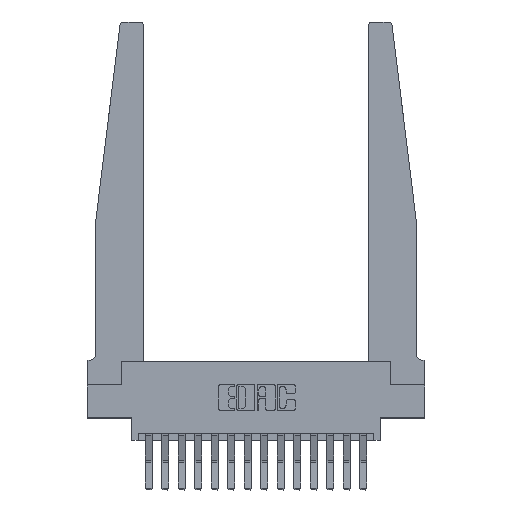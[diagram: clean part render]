
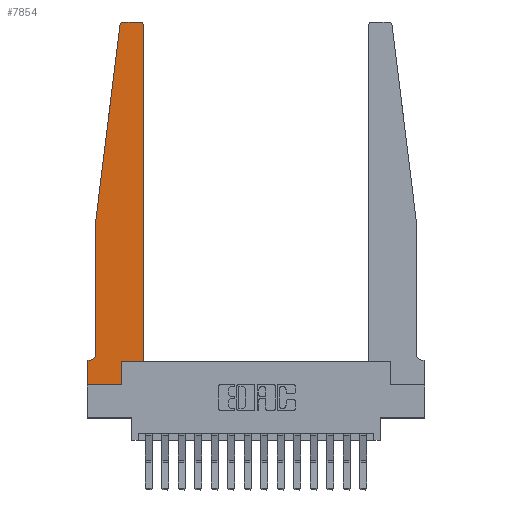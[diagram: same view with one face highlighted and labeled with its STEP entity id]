
A CAD part, top view. The second image highlights one B-rep face of the part: STEP entity #7854.
In plain terms, the highlighted planar face has unit normal (0, 0, 1).
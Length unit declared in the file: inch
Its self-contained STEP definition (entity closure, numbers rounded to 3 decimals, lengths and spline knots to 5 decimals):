
#316 = VERTEX_POINT ( 'NONE', #14830 ) ;
#393 = ORIENTED_EDGE ( 'NONE', *, *, #10516, .T. ) ;
#430 = AXIS2_PLACEMENT_3D ( 'NONE', #8690, #3119, #10266 ) ;
#656 = LINE ( 'NONE', #6327, #4585 ) ;
#957 = DIRECTION ( 'NONE',  ( 0., 1., 0. ) ) ;
#1023 = LINE ( 'NONE', #9667, #18153 ) ;
#1343 = VECTOR ( 'NONE', #957, 39.37008 ) ;
#1388 = EDGE_CURVE ( 'NONE', #12304, #15515, #12120, .T. ) ;
#1461 = DIRECTION ( 'NONE',  ( 0., 0., 1. ) ) ;
#1943 = DIRECTION ( 'NONE',  ( -1., 0., 0. ) ) ;
#2160 = VERTEX_POINT ( 'NONE', #16702 ) ;
#2281 = DIRECTION ( 'NONE',  ( 0., 0., 1. ) ) ;
#2345 = EDGE_CURVE ( 'NONE', #9796, #8731, #17068, .T. ) ;
#2382 = CARTESIAN_POINT ( 'NONE',  ( 0.015, 0.2375, 0.37 ) ) ;
#2872 = DIRECTION ( 'NONE',  ( 0., -1., 0. ) ) ;
#3025 = VERTEX_POINT ( 'NONE', #6925 ) ;
#3119 = DIRECTION ( 'NONE',  ( 0., 0., 1. ) ) ;
#3303 = VECTOR ( 'NONE', #7425, 39.37008 ) ;
#3355 = VECTOR ( 'NONE', #2872, 39.37008 ) ;
#3538 = ORIENTED_EDGE ( 'NONE', *, *, #6006, .T. ) ;
#3960 = EDGE_CURVE ( 'NONE', #8731, #12769, #9577, .T. ) ;
#4111 = ORIENTED_EDGE ( 'NONE', *, *, #2345, .T. ) ;
#4379 = CARTESIAN_POINT ( 'NONE',  ( 0.425, 0.18, 0.37 ) ) ;
#4579 = ORIENTED_EDGE ( 'NONE', *, *, #5078, .T. ) ;
#4585 = VECTOR ( 'NONE', #4944, 39.37008 ) ;
#4708 = EDGE_CURVE ( 'NONE', #18207, #9796, #1023, .T. ) ;
#4944 = DIRECTION ( 'NONE',  ( 0., -1., 0. ) ) ;
#5078 = EDGE_CURVE ( 'NONE', #13765, #14226, #15946, .T. ) ;
#5139 = VECTOR ( 'NONE', #16209, 39.37008 ) ;
#5142 = CARTESIAN_POINT ( 'NONE',  ( 0.2605, 0.18, 0.37 ) ) ;
#5202 = VECTOR ( 'NONE', #1943, 39.37008 ) ;
#5205 = DIRECTION ( 'NONE',  ( 1., 0., 0. ) ) ;
#5713 = ORIENTED_EDGE ( 'NONE', *, *, #1388, .T. ) ;
#5793 = ORIENTED_EDGE ( 'NONE', *, *, #13723, .T. ) ;
#6006 = EDGE_CURVE ( 'NONE', #3025, #12304, #656, .T. ) ;
#6063 = VECTOR ( 'NONE', #16045, 39.37008 ) ;
#6327 = CARTESIAN_POINT ( 'NONE',  ( 0.065, 1.25, 0.37 ) ) ;
#6925 = CARTESIAN_POINT ( 'NONE',  ( 0.065, 1.25, 0.37 ) ) ;
#7110 = ORIENTED_EDGE ( 'NONE', *, *, #15002, .T. ) ;
#7131 = FACE_OUTER_BOUND ( 'NONE', #17316, .T. ) ;
#7241 = EDGE_CURVE ( 'NONE', #14226, #18207, #9322, .T. ) ;
#7381 = ORIENTED_EDGE ( 'NONE', *, *, #7241, .T. ) ;
#7425 = DIRECTION ( 'NONE',  ( 0., 1., 0. ) ) ;
#7524 = VECTOR ( 'NONE', #10487, 39.37008 ) ;
#7686 = CARTESIAN_POINT ( 'NONE',  ( 0.065, 1.25, 0.37 ) ) ;
#7696 = CARTESIAN_POINT ( 'NONE',  ( 0., 0., 0.37 ) ) ;
#7854 = ADVANCED_FACE ( 'NONE', ( #7131 ), #8898, .T. ) ;
#7895 = CARTESIAN_POINT ( 'NONE',  ( 0.425, 2.72, 0.37 ) ) ;
#7953 = DIRECTION ( 'NONE',  ( 1., 0., 0. ) ) ;
#8147 = EDGE_CURVE ( 'NONE', #16716, #2160, #14038, .T. ) ;
#8156 = DIRECTION ( 'NONE',  ( -1., 0., 0. ) ) ;
#8446 = LINE ( 'NONE', #11208, #3355 ) ;
#8533 = CARTESIAN_POINT ( 'NONE',  ( 0., 0.1875, 0.37 ) ) ;
#8690 = CARTESIAN_POINT ( 'NONE',  ( 0.27653, 2.72, 0.37 ) ) ;
#8723 = CARTESIAN_POINT ( 'NONE',  ( 0.27653, 2.75, 0.37 ) ) ;
#8731 = VERTEX_POINT ( 'NONE', #7895 ) ;
#8736 = CARTESIAN_POINT ( 'NONE',  ( 0.065, 0.1875, 0.37 ) ) ;
#8898 = PLANE ( 'NONE',  #17351 ) ;
#9322 = LINE ( 'NONE', #5142, #1343 ) ;
#9577 = CIRCLE ( 'NONE', #12230, 0.03 ) ;
#9667 = CARTESIAN_POINT ( 'NONE',  ( 0.425, 0.18, 0.37 ) ) ;
#9796 = VERTEX_POINT ( 'NONE', #11247 ) ;
#9885 = CARTESIAN_POINT ( 'NONE',  ( 0.065, 0.2375, 0.37 ) ) ;
#10266 = DIRECTION ( 'NONE',  ( 1., 0., 0. ) ) ;
#10487 = DIRECTION ( 'NONE',  ( 1., 0., 0. ) ) ;
#10516 = EDGE_CURVE ( 'NONE', #2160, #3025, #16387, .T. ) ;
#10677 = CARTESIAN_POINT ( 'NONE',  ( 0., 0., 0.37 ) ) ;
#11208 = CARTESIAN_POINT ( 'NONE',  ( 0., 0., 0.37 ) ) ;
#11247 = CARTESIAN_POINT ( 'NONE',  ( 0.425, 0.18, 0.37 ) ) ;
#11561 = EDGE_CURVE ( 'NONE', #316, #13765, #8446, .T. ) ;
#11798 = ORIENTED_EDGE ( 'NONE', *, *, #8147, .T. ) ;
#12120 = CIRCLE ( 'NONE', #15682, 0.05 ) ;
#12219 = DIRECTION ( 'NONE',  ( 0., 0., -1. ) ) ;
#12230 = AXIS2_PLACEMENT_3D ( 'NONE', #14975, #2281, #7953 ) ;
#12304 = VERTEX_POINT ( 'NONE', #9885 ) ;
#12769 = VERTEX_POINT ( 'NONE', #14214 ) ;
#12771 = DIRECTION ( 'NONE',  ( 1., 0., 0. ) ) ;
#13065 = LINE ( 'NONE', #14641, #5202 ) ;
#13723 = EDGE_CURVE ( 'NONE', #15515, #316, #16229, .T. ) ;
#13765 = VERTEX_POINT ( 'NONE', #10677 ) ;
#14038 = CIRCLE ( 'NONE', #430, 0.03 ) ;
#14214 = CARTESIAN_POINT ( 'NONE',  ( 0.395, 2.75, 0.37 ) ) ;
#14226 = VERTEX_POINT ( 'NONE', #15742 ) ;
#14641 = CARTESIAN_POINT ( 'NONE',  ( 0.25, 2.75, 0.37 ) ) ;
#14713 = CARTESIAN_POINT ( 'NONE',  ( 0.015, 0.1875, 0.37 ) ) ;
#14830 = CARTESIAN_POINT ( 'NONE',  ( 0., 0.1875, 0.37 ) ) ;
#14975 = CARTESIAN_POINT ( 'NONE',  ( 0.395, 2.72, 0.37 ) ) ;
#15002 = EDGE_CURVE ( 'NONE', #12769, #16716, #13065, .T. ) ;
#15515 = VERTEX_POINT ( 'NONE', #14713 ) ;
#15682 = AXIS2_PLACEMENT_3D ( 'NONE', #2382, #12219, #8156 ) ;
#15742 = CARTESIAN_POINT ( 'NONE',  ( 0.2605, 0., 0.37 ) ) ;
#15946 = LINE ( 'NONE', #7696, #7524 ) ;
#16045 = DIRECTION ( 'NONE',  ( -1., 0., 0. ) ) ;
#16110 = ORIENTED_EDGE ( 'NONE', *, *, #11561, .T. ) ;
#16209 = DIRECTION ( 'NONE',  ( -0.122, -0.992, 0. ) ) ;
#16229 = LINE ( 'NONE', #8736, #6063 ) ;
#16387 = LINE ( 'NONE', #7686, #5139 ) ;
#16702 = CARTESIAN_POINT ( 'NONE',  ( 0.24675, 2.72367, 0.37 ) ) ;
#16716 = VERTEX_POINT ( 'NONE', #8723 ) ;
#17068 = LINE ( 'NONE', #4379, #3303 ) ;
#17316 = EDGE_LOOP ( 'NONE', ( #7110, #11798, #393, #3538, #5713, #5793, #16110, #4579, #7381, #18229, #4111, #18082 ) ) ;
#17351 = AXIS2_PLACEMENT_3D ( 'NONE', #8533, #1461, #12771 ) ;
#18082 = ORIENTED_EDGE ( 'NONE', *, *, #3960, .T. ) ;
#18153 = VECTOR ( 'NONE', #5205, 39.37008 ) ;
#18207 = VERTEX_POINT ( 'NONE', #18331 ) ;
#18229 = ORIENTED_EDGE ( 'NONE', *, *, #4708, .T. ) ;
#18331 = CARTESIAN_POINT ( 'NONE',  ( 0.2605, 0.18, 0.37 ) ) ;
